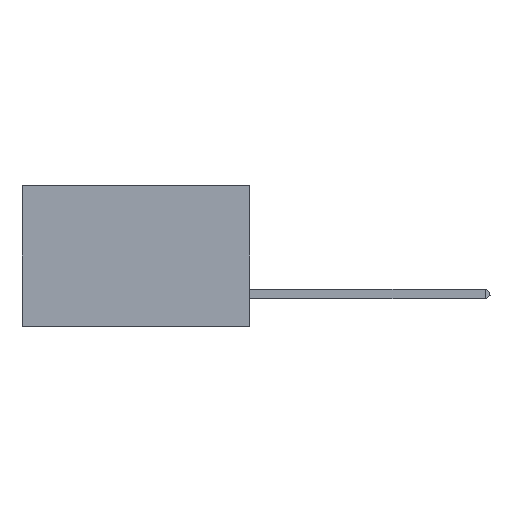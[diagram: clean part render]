
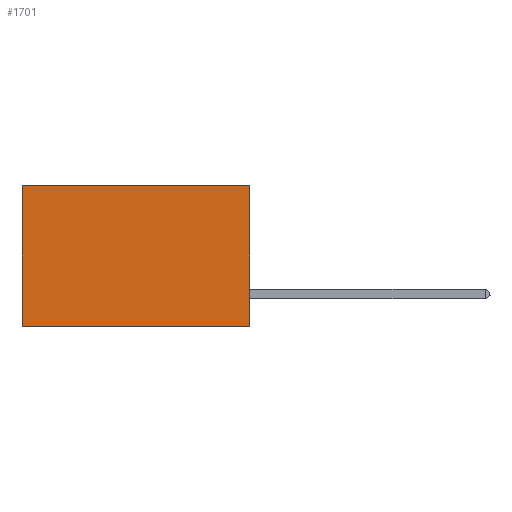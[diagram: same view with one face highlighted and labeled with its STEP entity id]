
A CAD part, left-side view. The second image highlights one B-rep face of the part: STEP entity #1701.
In plain terms, the highlighted planar face has unit normal (-1, 0, 0).
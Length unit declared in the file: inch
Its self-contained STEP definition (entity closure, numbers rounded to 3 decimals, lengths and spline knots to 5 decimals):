
#609 = VECTOR ( 'NONE', #12938, 39.37008 ) ;
#718 = VERTEX_POINT ( 'NONE', #8246 ) ;
#1288 = CARTESIAN_POINT ( 'NONE',  ( 0.2875, 0.6, 0. ) ) ;
#1516 = EDGE_CURVE ( 'NONE', #10247, #718, #9033, .T. ) ;
#1701 = ADVANCED_FACE ( 'NONE', ( #9895 ), #12320, .F. ) ;
#2307 = ORIENTED_EDGE ( 'NONE', *, *, #1516, .F. ) ;
#3898 = CARTESIAN_POINT ( 'NONE',  ( 0.2875, 0., 0. ) ) ;
#4075 = AXIS2_PLACEMENT_3D ( 'NONE', #6701, #4251, #13299 ) ;
#4251 = DIRECTION ( 'NONE',  ( 1., 0., 0. ) ) ;
#4328 = CARTESIAN_POINT ( 'NONE',  ( 0.2875, 0., -0.37 ) ) ;
#4500 = VECTOR ( 'NONE', #11261, 39.37008 ) ;
#6332 = EDGE_CURVE ( 'NONE', #718, #6415, #11480, .T. ) ;
#6415 = VERTEX_POINT ( 'NONE', #11384 ) ;
#6701 = CARTESIAN_POINT ( 'NONE',  ( 0.2875, 0., 0. ) ) ;
#7343 = CARTESIAN_POINT ( 'NONE',  ( 0.2875, 0., 0. ) ) ;
#8246 = CARTESIAN_POINT ( 'NONE',  ( 0.2875, 0., -0.37 ) ) ;
#8786 = VERTEX_POINT ( 'NONE', #14672 ) ;
#9033 = LINE ( 'NONE', #7343, #13607 ) ;
#9895 = FACE_OUTER_BOUND ( 'NONE', #14020, .T. ) ;
#10247 = VERTEX_POINT ( 'NONE', #13040 ) ;
#10485 = LINE ( 'NONE', #1288, #4500 ) ;
#10689 = ORIENTED_EDGE ( 'NONE', *, *, #6332, .F. ) ;
#10729 = ORIENTED_EDGE ( 'NONE', *, *, #14299, .T. ) ;
#11261 = DIRECTION ( 'NONE',  ( 0., 0., -1. ) ) ;
#11384 = CARTESIAN_POINT ( 'NONE',  ( 0.2875, 0.6, -0.37 ) ) ;
#11480 = LINE ( 'NONE', #4328, #13072 ) ;
#11565 = ORIENTED_EDGE ( 'NONE', *, *, #13604, .T. ) ;
#11868 = DIRECTION ( 'NONE',  ( 0., 0., -1. ) ) ;
#12320 = PLANE ( 'NONE',  #4075 ) ;
#12938 = DIRECTION ( 'NONE',  ( 0., 1., 0. ) ) ;
#13040 = CARTESIAN_POINT ( 'NONE',  ( 0.2875, 0., 0. ) ) ;
#13072 = VECTOR ( 'NONE', #14568, 39.37008 ) ;
#13299 = DIRECTION ( 'NONE',  ( 0., 0., -1. ) ) ;
#13604 = EDGE_CURVE ( 'NONE', #10247, #8786, #14065, .T. ) ;
#13607 = VECTOR ( 'NONE', #11868, 39.37008 ) ;
#14020 = EDGE_LOOP ( 'NONE', ( #10729, #10689, #2307, #11565 ) ) ;
#14065 = LINE ( 'NONE', #3898, #609 ) ;
#14299 = EDGE_CURVE ( 'NONE', #8786, #6415, #10485, .T. ) ;
#14568 = DIRECTION ( 'NONE',  ( 0., 1., 0. ) ) ;
#14672 = CARTESIAN_POINT ( 'NONE',  ( 0.2875, 0.6, 0. ) ) ;
